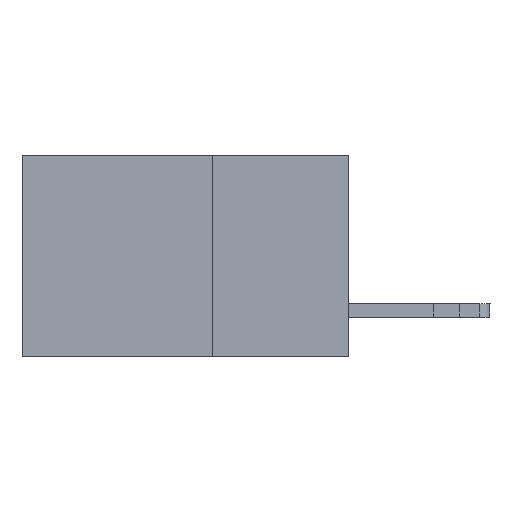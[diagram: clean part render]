
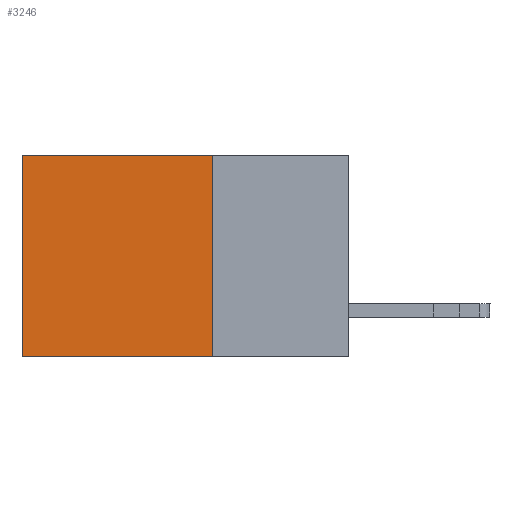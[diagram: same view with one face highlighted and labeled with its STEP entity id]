
A CAD part, left-side view. The second image highlights one B-rep face of the part: STEP entity #3246.
In plain terms, the highlighted planar face has unit normal (-1, 0, 0).
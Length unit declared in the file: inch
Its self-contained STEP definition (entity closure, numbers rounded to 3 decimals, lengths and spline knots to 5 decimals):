
#364 = EDGE_CURVE ( 'NONE', #11208, #1375, #7864, .T. ) ;
#1252 = FACE_OUTER_BOUND ( 'NONE', #7838, .T. ) ;
#1297 = EDGE_CURVE ( 'NONE', #1577, #12645, #12611, .T. ) ;
#1375 = VERTEX_POINT ( 'NONE', #2244 ) ;
#1577 = VERTEX_POINT ( 'NONE', #13145 ) ;
#2060 = VECTOR ( 'NONE', #6338, 39.37008 ) ;
#2244 = CARTESIAN_POINT ( 'NONE',  ( 0.2615, 0.6, -0.37 ) ) ;
#2601 = DIRECTION ( 'NONE',  ( 0., 1., 0. ) ) ;
#3195 = ORIENTED_EDGE ( 'NONE', *, *, #13106, .T. ) ;
#3240 = CARTESIAN_POINT ( 'NONE',  ( 0.2615, 0.25, -0.37 ) ) ;
#3246 = ADVANCED_FACE ( 'NONE', ( #1252 ), #9512, .F. ) ;
#3514 = EDGE_CURVE ( 'NONE', #1577, #11208, #8088, .T. ) ;
#4112 = DIRECTION ( 'NONE',  ( 1., 0., 0. ) ) ;
#4252 = DIRECTION ( 'NONE',  ( 0., 1., 0. ) ) ;
#4890 = VECTOR ( 'NONE', #4252, 39.37008 ) ;
#5111 = ORIENTED_EDGE ( 'NONE', *, *, #364, .F. ) ;
#5132 = VECTOR ( 'NONE', #5480, 39.37008 ) ;
#5310 = CARTESIAN_POINT ( 'NONE',  ( 0.2615, 0.25, 0. ) ) ;
#5480 = DIRECTION ( 'NONE',  ( 0., 0., -1. ) ) ;
#5716 = ORIENTED_EDGE ( 'NONE', *, *, #3514, .F. ) ;
#6103 = LINE ( 'NONE', #8551, #5132 ) ;
#6338 = DIRECTION ( 'NONE',  ( 0., 0., -1. ) ) ;
#6753 = CARTESIAN_POINT ( 'NONE',  ( 0.2615, 0.25, -0.37 ) ) ;
#7838 = EDGE_LOOP ( 'NONE', ( #3195, #5111, #5716, #10493 ) ) ;
#7864 = LINE ( 'NONE', #6753, #8859 ) ;
#8088 = LINE ( 'NONE', #8099, #2060 ) ;
#8099 = CARTESIAN_POINT ( 'NONE',  ( 0.2615, 0.25, -0.37 ) ) ;
#8551 = CARTESIAN_POINT ( 'NONE',  ( 0.2615, 0.6, -0.37 ) ) ;
#8859 = VECTOR ( 'NONE', #2601, 39.37008 ) ;
#9462 = DIRECTION ( 'NONE',  ( 0., 0., -1. ) ) ;
#9496 = CARTESIAN_POINT ( 'NONE',  ( 0.2615, 0.25, -0.37 ) ) ;
#9512 = PLANE ( 'NONE',  #12679 ) ;
#10493 = ORIENTED_EDGE ( 'NONE', *, *, #1297, .T. ) ;
#10797 = CARTESIAN_POINT ( 'NONE',  ( 0.2615, 0.6, 0. ) ) ;
#11208 = VERTEX_POINT ( 'NONE', #9496 ) ;
#12611 = LINE ( 'NONE', #5310, #4890 ) ;
#12645 = VERTEX_POINT ( 'NONE', #10797 ) ;
#12679 = AXIS2_PLACEMENT_3D ( 'NONE', #3240, #4112, #9462 ) ;
#13106 = EDGE_CURVE ( 'NONE', #12645, #1375, #6103, .T. ) ;
#13145 = CARTESIAN_POINT ( 'NONE',  ( 0.2615, 0.25, 0. ) ) ;
